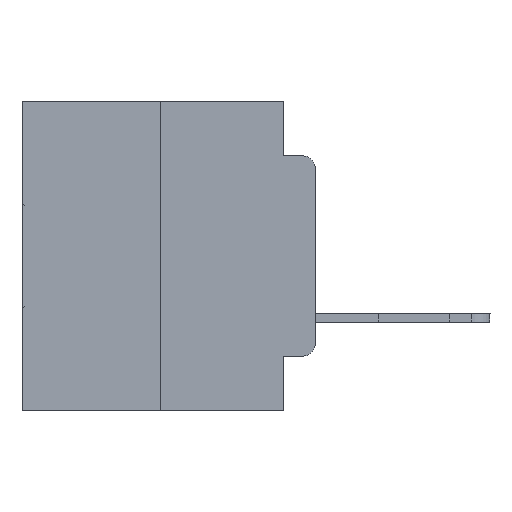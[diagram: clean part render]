
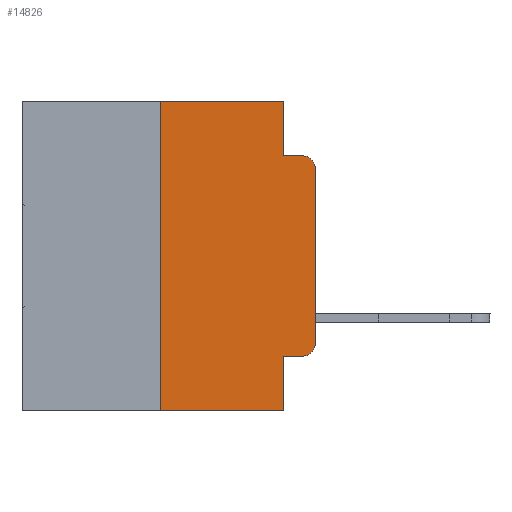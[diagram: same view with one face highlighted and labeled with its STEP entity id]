
A CAD part, left-side view. The second image highlights one B-rep face of the part: STEP entity #14826.
In plain terms, the highlighted planar face has unit normal (-1, 0, 0).
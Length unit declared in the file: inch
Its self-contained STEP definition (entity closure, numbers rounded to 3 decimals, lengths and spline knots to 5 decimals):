
#83 = VERTEX_POINT ( 'NONE', #24813 ) ;
#288 = EDGE_CURVE ( 'NONE', #25398, #24673, #12032, .T. ) ;
#449 = ORIENTED_EDGE ( 'NONE', *, *, #8650, .T. ) ;
#488 = CARTESIAN_POINT ( 'NONE',  ( 0., 0.051, -0.0885 ) ) ;
#1689 = EDGE_CURVE ( 'NONE', #3672, #83, #26139, .T. ) ;
#1743 = ORIENTED_EDGE ( 'NONE', *, *, #17923, .T. ) ;
#2785 = ORIENTED_EDGE ( 'NONE', *, *, #28363, .T. ) ;
#2850 = EDGE_LOOP ( 'NONE', ( #1743, #449, #24538, #20210, #27556, #3581, #2785, #11926, #3821, #19567 ) ) ;
#3051 = CARTESIAN_POINT ( 'NONE',  ( 0., 0., 0. ) ) ;
#3581 = ORIENTED_EDGE ( 'NONE', *, *, #4310, .F. ) ;
#3672 = VERTEX_POINT ( 'NONE', #6389 ) ;
#3677 = VECTOR ( 'NONE', #24246, 39.37008 ) ;
#3821 = ORIENTED_EDGE ( 'NONE', *, *, #1689, .T. ) ;
#3845 = DIRECTION ( 'NONE',  ( 0., -1., 0. ) ) ;
#4310 = EDGE_CURVE ( 'NONE', #26045, #19676, #23682, .T. ) ;
#4614 = EDGE_CURVE ( 'NONE', #3672, #24942, #9520, .T. ) ;
#6264 = CARTESIAN_POINT ( 'NONE',  ( 0., 0.051, -0.4115 ) ) ;
#6389 = CARTESIAN_POINT ( 'NONE',  ( 0., 0.051, -0.4115 ) ) ;
#6536 = CARTESIAN_POINT ( 'NONE',  ( 0., 0.02, -0.0885 ) ) ;
#6690 = VECTOR ( 'NONE', #19191, 39.37008 ) ;
#6745 = PLANE ( 'NONE',  #27126 ) ;
#7137 = CARTESIAN_POINT ( 'NONE',  ( 0., 0.051, 0. ) ) ;
#7633 = AXIS2_PLACEMENT_3D ( 'NONE', #10379, #28594, #8104 ) ;
#7879 = CARTESIAN_POINT ( 'NONE',  ( 0., 0.25, 0. ) ) ;
#8104 = DIRECTION ( 'NONE',  ( 0., 0., -1. ) ) ;
#8650 = EDGE_CURVE ( 'NONE', #9457, #9357, #28049, .T. ) ;
#9357 = VERTEX_POINT ( 'NONE', #6536 ) ;
#9457 = VERTEX_POINT ( 'NONE', #20605 ) ;
#9472 = CARTESIAN_POINT ( 'NONE',  ( 0., 0.051, -0.0885 ) ) ;
#9520 = LINE ( 'NONE', #17915, #22631 ) ;
#9600 = CARTESIAN_POINT ( 'NONE',  ( 0., 0.02, -0.3915 ) ) ;
#10140 = CARTESIAN_POINT ( 'NONE',  ( 0., 0.051, -0.5 ) ) ;
#10379 = CARTESIAN_POINT ( 'NONE',  ( 0., 0.02, -0.1085 ) ) ;
#11926 = ORIENTED_EDGE ( 'NONE', *, *, #4614, .F. ) ;
#12032 = LINE ( 'NONE', #7137, #26558 ) ;
#13604 = LINE ( 'NONE', #3051, #3677 ) ;
#13984 = DIRECTION ( 'NONE',  ( 0., -1., 0. ) ) ;
#14099 = DIRECTION ( 'NONE',  ( 1., 0., 0. ) ) ;
#14155 = LINE ( 'NONE', #14573, #6690 ) ;
#14573 = CARTESIAN_POINT ( 'NONE',  ( 0., 0.473, 0. ) ) ;
#14826 = ADVANCED_FACE ( 'NONE', ( #18120 ), #6745, .F. ) ;
#16454 = CARTESIAN_POINT ( 'NONE',  ( 0., 0.051, 0. ) ) ;
#16479 = DIRECTION ( 'NONE',  ( 0., 0., -1. ) ) ;
#17056 = CARTESIAN_POINT ( 'NONE',  ( 0., 0.25, 0. ) ) ;
#17231 = VERTEX_POINT ( 'NONE', #23673 ) ;
#17302 = VECTOR ( 'NONE', #3845, 39.37008 ) ;
#17425 = LINE ( 'NONE', #488, #19182 ) ;
#17779 = EDGE_CURVE ( 'NONE', #83, #17231, #24596, .T. ) ;
#17915 = CARTESIAN_POINT ( 'NONE',  ( 0., 0.051, 0. ) ) ;
#17923 = EDGE_CURVE ( 'NONE', #17231, #9457, #13604, .T. ) ;
#18120 = FACE_OUTER_BOUND ( 'NONE', #2850, .T. ) ;
#19182 = VECTOR ( 'NONE', #13984, 39.37008 ) ;
#19191 = DIRECTION ( 'NONE',  ( 0., -1., 0. ) ) ;
#19265 = DIRECTION ( 'NONE',  ( 0., 0., 1. ) ) ;
#19383 = AXIS2_PLACEMENT_3D ( 'NONE', #9600, #25244, #25523 ) ;
#19567 = ORIENTED_EDGE ( 'NONE', *, *, #17779, .T. ) ;
#19676 = VERTEX_POINT ( 'NONE', #17056 ) ;
#20210 = ORIENTED_EDGE ( 'NONE', *, *, #288, .F. ) ;
#20230 = CARTESIAN_POINT ( 'NONE',  ( 0., 0.473, 0. ) ) ;
#20605 = CARTESIAN_POINT ( 'NONE',  ( 0., 0., -0.1085 ) ) ;
#21380 = LINE ( 'NONE', #27933, #26339 ) ;
#21947 = EDGE_CURVE ( 'NONE', #19676, #25398, #14155, .T. ) ;
#22065 = CARTESIAN_POINT ( 'NONE',  ( 0., 0.25, -0.5 ) ) ;
#22631 = VECTOR ( 'NONE', #24655, 39.37008 ) ;
#23011 = DIRECTION ( 'NONE',  ( 0., 0., -1. ) ) ;
#23673 = CARTESIAN_POINT ( 'NONE',  ( 0., 0., -0.3915 ) ) ;
#23682 = LINE ( 'NONE', #7879, #24782 ) ;
#24246 = DIRECTION ( 'NONE',  ( 0., 0., 1. ) ) ;
#24538 = ORIENTED_EDGE ( 'NONE', *, *, #25782, .F. ) ;
#24596 = CIRCLE ( 'NONE', #19383, 0.02 ) ;
#24655 = DIRECTION ( 'NONE',  ( 0., 0., -1. ) ) ;
#24673 = VERTEX_POINT ( 'NONE', #9472 ) ;
#24782 = VECTOR ( 'NONE', #19265, 39.37008 ) ;
#24813 = CARTESIAN_POINT ( 'NONE',  ( 0., 0.02, -0.4115 ) ) ;
#24942 = VERTEX_POINT ( 'NONE', #10140 ) ;
#25244 = DIRECTION ( 'NONE',  ( -1., 0., 0. ) ) ;
#25398 = VERTEX_POINT ( 'NONE', #16454 ) ;
#25523 = DIRECTION ( 'NONE',  ( 0., 0., -1. ) ) ;
#25782 = EDGE_CURVE ( 'NONE', #24673, #9357, #17425, .T. ) ;
#26045 = VERTEX_POINT ( 'NONE', #22065 ) ;
#26139 = LINE ( 'NONE', #6264, #17302 ) ;
#26261 = DIRECTION ( 'NONE',  ( 0., -1., 0. ) ) ;
#26339 = VECTOR ( 'NONE', #26261, 39.37008 ) ;
#26558 = VECTOR ( 'NONE', #23011, 39.37008 ) ;
#27126 = AXIS2_PLACEMENT_3D ( 'NONE', #20230, #14099, #16479 ) ;
#27556 = ORIENTED_EDGE ( 'NONE', *, *, #21947, .F. ) ;
#27933 = CARTESIAN_POINT ( 'NONE',  ( 0., 0.473, -0.5 ) ) ;
#28049 = CIRCLE ( 'NONE', #7633, 0.02 ) ;
#28363 = EDGE_CURVE ( 'NONE', #26045, #24942, #21380, .T. ) ;
#28594 = DIRECTION ( 'NONE',  ( -1., 0., 0. ) ) ;
